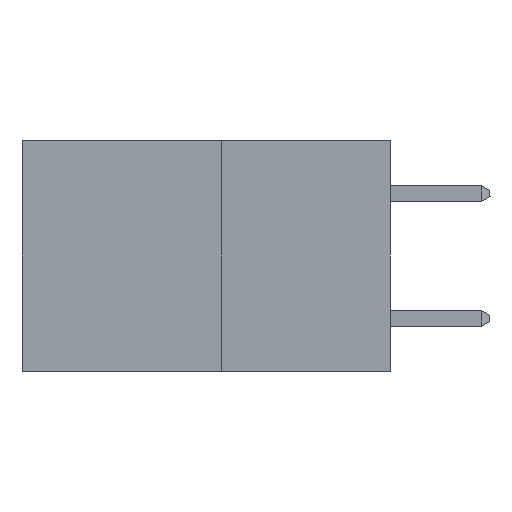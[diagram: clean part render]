
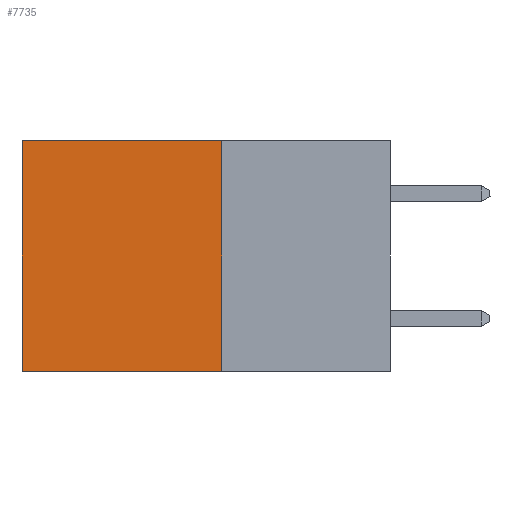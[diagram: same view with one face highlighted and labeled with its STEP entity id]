
A CAD part, left-side view. The second image highlights one B-rep face of the part: STEP entity #7735.
In plain terms, the highlighted planar face has unit normal (-1, 0, 0).
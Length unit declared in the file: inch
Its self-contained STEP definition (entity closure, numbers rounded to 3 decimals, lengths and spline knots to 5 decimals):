
#554 = ORIENTED_EDGE ( 'NONE', *, *, #13095, .T. ) ;
#557 = ORIENTED_EDGE ( 'NONE', *, *, #11487, .F. ) ;
#699 = CARTESIAN_POINT ( 'NONE',  ( 0.277, 0.59, 0. ) ) ;
#717 = ORIENTED_EDGE ( 'NONE', *, *, #11843, .F. ) ;
#1035 = VERTEX_POINT ( 'NONE', #9315 ) ;
#1097 = ORIENTED_EDGE ( 'NONE', *, *, #1881, .T. ) ;
#1107 = AXIS2_PLACEMENT_3D ( 'NONE', #7040, #8148, #5383 ) ;
#1149 = LINE ( 'NONE', #15059, #13707 ) ;
#1326 = CARTESIAN_POINT ( 'NONE',  ( 0.277, 0.27, 0. ) ) ;
#1881 = EDGE_CURVE ( 'NONE', #6985, #15399, #15118, .T. ) ;
#3030 = VECTOR ( 'NONE', #3903, 39.37008 ) ;
#3903 = DIRECTION ( 'NONE',  ( 0., 0., -1. ) ) ;
#4002 = CARTESIAN_POINT ( 'NONE',  ( 0.277, 0.59, -0.37 ) ) ;
#5171 = VERTEX_POINT ( 'NONE', #9514 ) ;
#5231 = VECTOR ( 'NONE', #12567, 39.37008 ) ;
#5383 = DIRECTION ( 'NONE',  ( 0., 0., -1. ) ) ;
#6304 = LINE ( 'NONE', #4002, #3030 ) ;
#6985 = VERTEX_POINT ( 'NONE', #8118 ) ;
#7040 = CARTESIAN_POINT ( 'NONE',  ( 0.277, 0.27, -0.37 ) ) ;
#7735 = ADVANCED_FACE ( 'NONE', ( #12304 ), #8001, .F. ) ;
#8001 = PLANE ( 'NONE',  #1107 ) ;
#8118 = CARTESIAN_POINT ( 'NONE',  ( 0.277, 0.27, 0. ) ) ;
#8148 = DIRECTION ( 'NONE',  ( 1., 0., 0. ) ) ;
#9092 = VECTOR ( 'NONE', #13685, 39.37008 ) ;
#9315 = CARTESIAN_POINT ( 'NONE',  ( 0.277, 0.59, -0.37 ) ) ;
#9514 = CARTESIAN_POINT ( 'NONE',  ( 0.277, 0.27, -0.37 ) ) ;
#11262 = LINE ( 'NONE', #12568, #5231 ) ;
#11299 = EDGE_LOOP ( 'NONE', ( #554, #557, #717, #1097 ) ) ;
#11487 = EDGE_CURVE ( 'NONE', #5171, #1035, #1149, .T. ) ;
#11843 = EDGE_CURVE ( 'NONE', #6985, #5171, #11262, .T. ) ;
#12304 = FACE_OUTER_BOUND ( 'NONE', #11299, .T. ) ;
#12567 = DIRECTION ( 'NONE',  ( 0., 0., -1. ) ) ;
#12568 = CARTESIAN_POINT ( 'NONE',  ( 0.277, 0.27, -0.37 ) ) ;
#13095 = EDGE_CURVE ( 'NONE', #15399, #1035, #6304, .T. ) ;
#13685 = DIRECTION ( 'NONE',  ( 0., 1., 0. ) ) ;
#13707 = VECTOR ( 'NONE', #15037, 39.37008 ) ;
#15037 = DIRECTION ( 'NONE',  ( 0., 1., 0. ) ) ;
#15059 = CARTESIAN_POINT ( 'NONE',  ( 0.277, 0.27, -0.37 ) ) ;
#15118 = LINE ( 'NONE', #1326, #9092 ) ;
#15399 = VERTEX_POINT ( 'NONE', #699 ) ;
